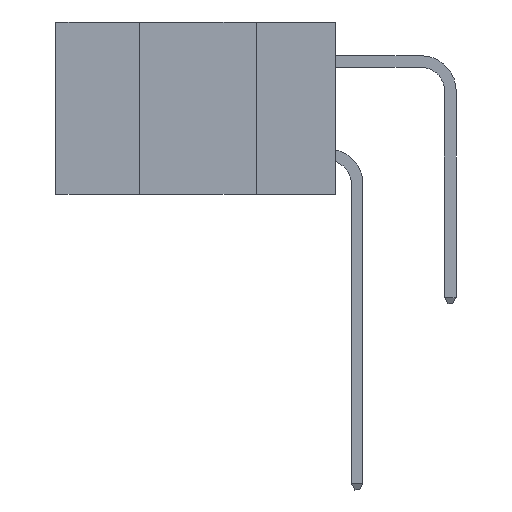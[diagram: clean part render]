
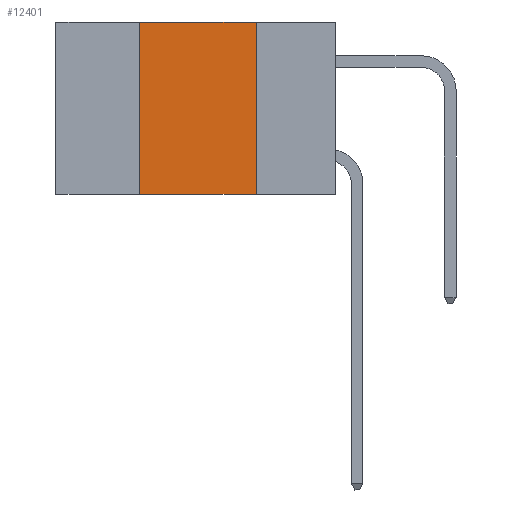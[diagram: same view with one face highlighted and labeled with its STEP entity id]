
A CAD part, left-side view. The second image highlights one B-rep face of the part: STEP entity #12401.
In plain terms, the highlighted planar face has unit normal (-1, 0, 0).
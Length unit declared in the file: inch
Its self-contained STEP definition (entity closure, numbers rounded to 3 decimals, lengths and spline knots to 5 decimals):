
#35 = EDGE_LOOP ( 'NONE', ( #1124, #13221, #1431, #11716 ) ) ;
#396 = DIRECTION ( 'NONE',  ( 1., 0., 0. ) ) ;
#543 = CARTESIAN_POINT ( 'NONE',  ( 0., 0.6, 0. ) ) ;
#1124 = ORIENTED_EDGE ( 'NONE', *, *, #10724, .F. ) ;
#1279 = VECTOR ( 'NONE', #2921, 39.37008 ) ;
#1431 = ORIENTED_EDGE ( 'NONE', *, *, #14240, .F. ) ;
#1868 = DIRECTION ( 'NONE',  ( 0., -1., 0. ) ) ;
#2921 = DIRECTION ( 'NONE',  ( 0., 0., -1. ) ) ;
#2955 = PLANE ( 'NONE',  #6467 ) ;
#3313 = VERTEX_POINT ( 'NONE', #7989 ) ;
#4123 = VERTEX_POINT ( 'NONE', #7079 ) ;
#4539 = CARTESIAN_POINT ( 'NONE',  ( 0., 0.42, -0.37 ) ) ;
#4786 = VERTEX_POINT ( 'NONE', #4539 ) ;
#6274 = CARTESIAN_POINT ( 'NONE',  ( 0., 0.17, 0. ) ) ;
#6467 = AXIS2_PLACEMENT_3D ( 'NONE', #9138, #396, #12713 ) ;
#7079 = CARTESIAN_POINT ( 'NONE',  ( 0., 0.42, 0. ) ) ;
#7360 = LINE ( 'NONE', #543, #8883 ) ;
#7989 = CARTESIAN_POINT ( 'NONE',  ( 0., 0.17, 0. ) ) ;
#8155 = LINE ( 'NONE', #14191, #13222 ) ;
#8296 = DIRECTION ( 'NONE',  ( 0., 0., 1. ) ) ;
#8389 = LINE ( 'NONE', #13849, #12571 ) ;
#8730 = EDGE_CURVE ( 'NONE', #4786, #11798, #8155, .T. ) ;
#8883 = VECTOR ( 'NONE', #11557, 39.37008 ) ;
#9138 = CARTESIAN_POINT ( 'NONE',  ( 0., 0.6, 0. ) ) ;
#9503 = CARTESIAN_POINT ( 'NONE',  ( 0., 0.17, -0.37 ) ) ;
#9653 = LINE ( 'NONE', #6274, #1279 ) ;
#10512 = FACE_OUTER_BOUND ( 'NONE', #35, .T. ) ;
#10724 = EDGE_CURVE ( 'NONE', #3313, #11798, #9653, .T. ) ;
#11557 = DIRECTION ( 'NONE',  ( 0., -1., 0. ) ) ;
#11716 = ORIENTED_EDGE ( 'NONE', *, *, #8730, .T. ) ;
#11798 = VERTEX_POINT ( 'NONE', #9503 ) ;
#12401 = ADVANCED_FACE ( 'NONE', ( #10512 ), #2955, .F. ) ;
#12571 = VECTOR ( 'NONE', #8296, 39.37008 ) ;
#12713 = DIRECTION ( 'NONE',  ( 0., 0., -1. ) ) ;
#13221 = ORIENTED_EDGE ( 'NONE', *, *, #14316, .F. ) ;
#13222 = VECTOR ( 'NONE', #1868, 39.37008 ) ;
#13849 = CARTESIAN_POINT ( 'NONE',  ( 0., 0.42, 0. ) ) ;
#14191 = CARTESIAN_POINT ( 'NONE',  ( 0., 0.6, -0.37 ) ) ;
#14240 = EDGE_CURVE ( 'NONE', #4786, #4123, #8389, .T. ) ;
#14316 = EDGE_CURVE ( 'NONE', #4123, #3313, #7360, .T. ) ;
